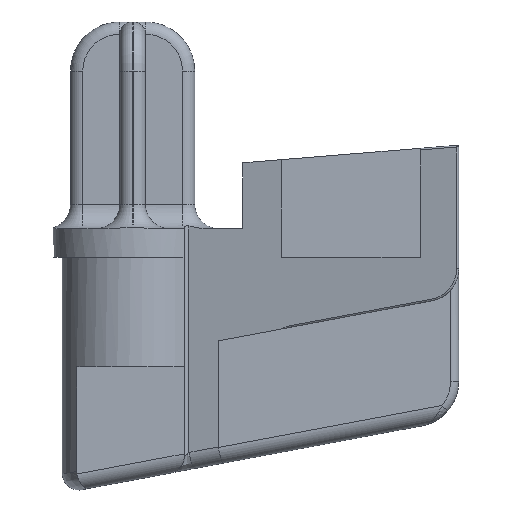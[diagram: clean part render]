
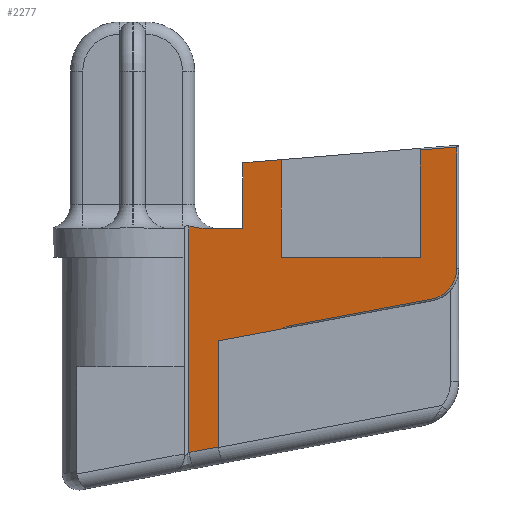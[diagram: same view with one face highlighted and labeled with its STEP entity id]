
A CAD part, left-side view. The second image highlights one B-rep face of the part: STEP entity #2277.
In plain terms, the highlighted planar face has unit normal (-0.982, 0.187, 0).
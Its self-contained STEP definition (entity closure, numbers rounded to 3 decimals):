
#47=PLANE('',#2481);
#85=B_SPLINE_CURVE_WITH_KNOTS('',3,(#3646,#3647,#3648,#3649,#3650,#3651,
#3652,#3653,#3654),.UNSPECIFIED.,.F.,.F.,(4,1,1,1,1,1,4),(0.,0.025,
0.042,0.05,0.054,0.057,
0.059),.UNSPECIFIED.);
#103=B_SPLINE_CURVE_WITH_KNOTS('',3,(#4231,#4232,#4233,#4234,#4235,#4236),
 .UNSPECIFIED.,.F.,.F.,(4,2,4),(-1.566,-1.521,-1.462),
 .UNSPECIFIED.);
#115=ELLIPSE('',#2399,1.934,1.9);
#162=LINE('',#3446,#340);
#165=LINE('',#3456,#343);
#166=LINE('',#3493,#344);
#190=LINE('',#3715,#368);
#203=LINE('',#3882,#381);
#228=LINE('',#4163,#406);
#229=LINE('',#4166,#407);
#236=LINE('',#4220,#414);
#237=LINE('',#4222,#415);
#238=LINE('',#4224,#416);
#239=LINE('',#4226,#417);
#240=LINE('',#4228,#418);
#241=LINE('',#4230,#419);
#340=VECTOR('',#2697,10.);
#343=VECTOR('',#2706,10.);
#344=VECTOR('',#2715,10.);
#368=VECTOR('',#2765,10.);
#381=VECTOR('',#2818,10.);
#406=VECTOR('',#2917,10.);
#407=VECTOR('',#2920,10.);
#414=VECTOR('',#2945,10.);
#415=VECTOR('',#2946,10.);
#416=VECTOR('',#2947,10.);
#417=VECTOR('',#2948,10.);
#418=VECTOR('',#2949,10.);
#419=VECTOR('',#2950,10.);
#625=FACE_OUTER_BOUND('',#764,.T.);
#764=EDGE_LOOP('',(#1798,#1799,#1800,#1801,#1802,#1803,#1804,#1805,#1806,
#1807,#1808,#1809,#1810,#1811,#1812,#1813));
#959=VERTEX_POINT('',#3374);
#973=VERTEX_POINT('',#3444);
#974=VERTEX_POINT('',#3449);
#977=VERTEX_POINT('',#3454);
#979=VERTEX_POINT('',#3488);
#985=VERTEX_POINT('',#3645);
#1002=VERTEX_POINT('',#3714);
#1024=VERTEX_POINT('',#3881);
#1057=VERTEX_POINT('',#4159);
#1058=VERTEX_POINT('',#4165);
#1064=VERTEX_POINT('',#4219);
#1065=VERTEX_POINT('',#4221);
#1066=VERTEX_POINT('',#4223);
#1067=VERTEX_POINT('',#4225);
#1068=VERTEX_POINT('',#4227);
#1069=VERTEX_POINT('',#4229);
#1191=EDGE_CURVE('',#973,#959,#162,.T.);
#1196=EDGE_CURVE('',#977,#974,#165,.T.);
#1198=EDGE_CURVE('',#979,#977,#115,.T.);
#1200=EDGE_CURVE('',#959,#979,#166,.T.);
#1209=EDGE_CURVE('',#974,#985,#85,.T.);
#1234=EDGE_CURVE('',#1002,#985,#190,.T.);
#1265=EDGE_CURVE('',#1024,#1002,#203,.T.);
#1320=EDGE_CURVE('',#1024,#1057,#228,.T.);
#1321=EDGE_CURVE('',#1057,#1058,#229,.T.);
#1334=EDGE_CURVE('',#1064,#973,#236,.T.);
#1335=EDGE_CURVE('',#1065,#1064,#237,.T.);
#1336=EDGE_CURVE('',#1065,#1066,#238,.T.);
#1337=EDGE_CURVE('',#1067,#1066,#239,.T.);
#1338=EDGE_CURVE('',#1068,#1067,#240,.T.);
#1339=EDGE_CURVE('',#1069,#1068,#241,.T.);
#1340=EDGE_CURVE('',#1069,#1058,#103,.F.);
#1798=ORIENTED_EDGE('',*,*,#1191,.F.);
#1799=ORIENTED_EDGE('',*,*,#1334,.F.);
#1800=ORIENTED_EDGE('',*,*,#1335,.F.);
#1801=ORIENTED_EDGE('',*,*,#1336,.T.);
#1802=ORIENTED_EDGE('',*,*,#1337,.F.);
#1803=ORIENTED_EDGE('',*,*,#1338,.F.);
#1804=ORIENTED_EDGE('',*,*,#1339,.F.);
#1805=ORIENTED_EDGE('',*,*,#1340,.T.);
#1806=ORIENTED_EDGE('',*,*,#1321,.F.);
#1807=ORIENTED_EDGE('',*,*,#1320,.F.);
#1808=ORIENTED_EDGE('',*,*,#1265,.T.);
#1809=ORIENTED_EDGE('',*,*,#1234,.T.);
#1810=ORIENTED_EDGE('',*,*,#1209,.F.);
#1811=ORIENTED_EDGE('',*,*,#1196,.F.);
#1812=ORIENTED_EDGE('',*,*,#1198,.F.);
#1813=ORIENTED_EDGE('',*,*,#1200,.F.);
#2277=ADVANCED_FACE('',(#625),#47,.T.);
#2399=AXIS2_PLACEMENT_3D('',#3490,#2709,#2710);
#2481=AXIS2_PLACEMENT_3D('',#4218,#2943,#2944);
#2697=DIRECTION('',(-0.186,-0.979,0.08));
#2706=DIRECTION('',(0.184,0.966,-0.181));
#2709=DIRECTION('center_axis',(0.982,-0.187,0.));
#2710=DIRECTION('ref_axis',(-0.187,-0.982,0.));
#2715=DIRECTION('',(0.,0.,-1.));
#2765=DIRECTION('',(-0.184,-0.966,0.181));
#2818=DIRECTION('',(0.,0.,1.));
#2917=DIRECTION('',(0.184,0.966,-0.181));
#2920=DIRECTION('',(0.,0.,1.));
#2943=DIRECTION('center_axis',(-0.982,0.187,0.));
#2944=DIRECTION('ref_axis',(-0.187,-0.982,0.));
#2945=DIRECTION('',(0.,0.,1.));
#2946=DIRECTION('',(-0.187,-0.982,0.));
#2947=DIRECTION('',(0.,0.,1.));
#2948=DIRECTION('',(-0.186,-0.979,0.08));
#2949=DIRECTION('',(0.,0.,1.));
#2950=DIRECTION('',(-0.187,-0.982,0.));
#3374=CARTESIAN_POINT('',(-10.777,9.919,6.754));
#3444=CARTESIAN_POINT('',(-10.352,12.15,6.572));
#3446=CARTESIAN_POINT('',(-8.171,23.603,5.639));
#3449=CARTESIAN_POINT('',(-8.848,20.049,-4.168));
#3454=CARTESIAN_POINT('',(-10.482,11.468,-2.558));
#3456=CARTESIAN_POINT('',(-10.572,10.998,-2.47));
#3488=CARTESIAN_POINT('',(-10.777,9.919,-0.69));
#3490=CARTESIAN_POINT('Origin',(-10.416,11.819,-0.69));
#3493=CARTESIAN_POINT('',(-10.777,9.919,0.));
#3645=CARTESIAN_POINT('',(-8.748,20.574,-4.371));
#3646=CARTESIAN_POINT('Ctrl Pts',(-8.848,20.049,-4.168));
#3647=CARTESIAN_POINT('Ctrl Pts',(-8.833,20.13,-4.183));
#3648=CARTESIAN_POINT('Ctrl Pts',(-8.807,20.264,-4.214));
#3649=CARTESIAN_POINT('Ctrl Pts',(-8.777,20.421,-4.265));
#3650=CARTESIAN_POINT('Ctrl Pts',(-8.761,20.509,-4.305));
#3651=CARTESIAN_POINT('Ctrl Pts',(-8.753,20.55,-4.331));
#3652=CARTESIAN_POINT('Ctrl Pts',(-8.749,20.57,-4.351));
#3653=CARTESIAN_POINT('Ctrl Pts',(-8.748,20.575,-4.365));
#3654=CARTESIAN_POINT('Ctrl Pts',(-8.748,20.574,-4.371));
#3714=CARTESIAN_POINT('',(-8.,24.504,-5.109));
#3715=CARTESIAN_POINT('',(-9.645,15.864,-3.488));
#3881=CARTESIAN_POINT('',(-8.,24.504,-11.596));
#3882=CARTESIAN_POINT('',(-8.,24.504,-4.945));
#4159=CARTESIAN_POINT('',(-7.657,26.303,-11.933));
#4163=CARTESIAN_POINT('',(-8.394,22.435,-11.207));
#4165=CARTESIAN_POINT('',(-7.657,26.303,1.919));
#4166=CARTESIAN_POINT('',(-7.657,26.303,0.875));
#4218=CARTESIAN_POINT('Origin',(-10.352,12.15,0.));
#4219=CARTESIAN_POINT('',(-10.352,12.15,0.));
#4220=CARTESIAN_POINT('',(-10.352,12.15,3.559));
#4221=CARTESIAN_POINT('',(-8.734,20.65,0.));
#4222=CARTESIAN_POINT('',(-8.661,21.03,0.));
#4223=CARTESIAN_POINT('',(-8.734,20.65,5.978));
#4224=CARTESIAN_POINT('',(-8.734,20.65,0.));
#4225=CARTESIAN_POINT('',(-8.286,23.,5.787));
#4226=CARTESIAN_POINT('',(-7.167,28.88,5.308));
#4227=CARTESIAN_POINT('',(-8.286,23.,1.75));
#4228=CARTESIAN_POINT('',(-8.286,23.,0.));
#4229=CARTESIAN_POINT('',(-7.86,25.238,1.75));
#4230=CARTESIAN_POINT('',(-6.125,34.35,1.75));
#4231=CARTESIAN_POINT('Ctrl Pts',(-7.657,26.303,1.919));
#4232=CARTESIAN_POINT('Ctrl Pts',(-7.687,26.146,1.883));
#4233=CARTESIAN_POINT('Ctrl Pts',(-7.717,25.991,1.845));
#4234=CARTESIAN_POINT('Ctrl Pts',(-7.78,25.658,1.779));
#4235=CARTESIAN_POINT('Ctrl Pts',(-7.824,25.43,1.75));
#4236=CARTESIAN_POINT('Ctrl Pts',(-7.86,25.238,1.75));
